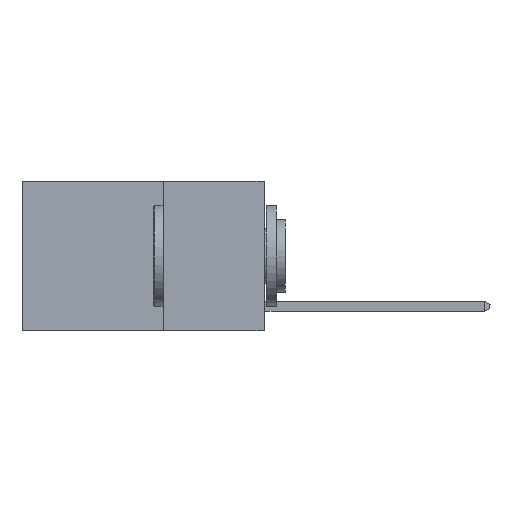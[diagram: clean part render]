
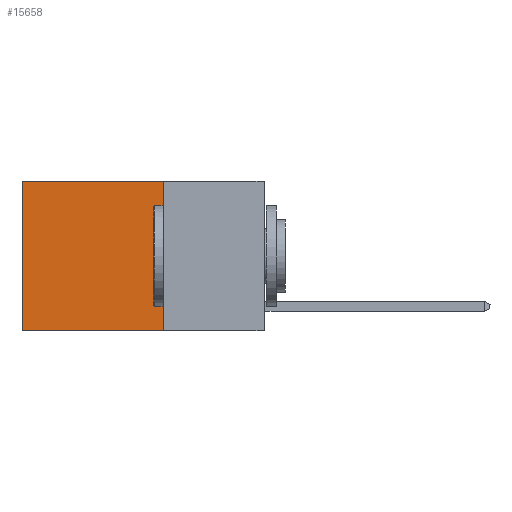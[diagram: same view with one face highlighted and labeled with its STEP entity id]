
A CAD part, left-side view. The second image highlights one B-rep face of the part: STEP entity #15658.
In plain terms, the highlighted planar face has unit normal (-1, 0, 0).
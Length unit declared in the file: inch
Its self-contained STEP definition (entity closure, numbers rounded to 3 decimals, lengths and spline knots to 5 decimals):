
#1158 = DIRECTION ( 'NONE',  ( 0., 1., 0. ) ) ;
#2014 = ORIENTED_EDGE ( 'NONE', *, *, #3535, .T. ) ;
#2140 = LINE ( 'NONE', #5242, #6266 ) ;
#3189 = LINE ( 'NONE', #15105, #11526 ) ;
#3535 = EDGE_CURVE ( 'NONE', #20967, #20801, #2140, .T. ) ;
#3891 = VECTOR ( 'NONE', #13167, 39.37008 ) ;
#5242 = CARTESIAN_POINT ( 'NONE',  ( 0.2625, 0.6, 0. ) ) ;
#5927 = ORIENTED_EDGE ( 'NONE', *, *, #17753, .F. ) ;
#6100 = ORIENTED_EDGE ( 'NONE', *, *, #11430, .T. ) ;
#6115 = FACE_OUTER_BOUND ( 'NONE', #7543, .T. ) ;
#6266 = VECTOR ( 'NONE', #21471, 39.37008 ) ;
#7543 = EDGE_LOOP ( 'NONE', ( #2014, #5927, #8857, #6100 ) ) ;
#8857 = ORIENTED_EDGE ( 'NONE', *, *, #12803, .F. ) ;
#9450 = VERTEX_POINT ( 'NONE', #15922 ) ;
#11430 = EDGE_CURVE ( 'NONE', #22941, #20967, #3189, .T. ) ;
#11526 = VECTOR ( 'NONE', #1158, 39.37008 ) ;
#12537 = VECTOR ( 'NONE', #27641, 39.37008 ) ;
#12803 = EDGE_CURVE ( 'NONE', #22941, #9450, #15642, .T. ) ;
#13167 = DIRECTION ( 'NONE',  ( 0., 0., -1. ) ) ;
#13517 = DIRECTION ( 'NONE',  ( 0., 0., -1. ) ) ;
#15105 = CARTESIAN_POINT ( 'NONE',  ( 0.2625, 0.25, 0. ) ) ;
#15642 = LINE ( 'NONE', #24773, #3891 ) ;
#15658 = ADVANCED_FACE ( 'NONE', ( #6115 ), #30054, .F. ) ;
#15907 = AXIS2_PLACEMENT_3D ( 'NONE', #25119, #25570, #13517 ) ;
#15922 = CARTESIAN_POINT ( 'NONE',  ( 0.2625, 0.25, -0.37 ) ) ;
#17753 = EDGE_CURVE ( 'NONE', #9450, #20801, #23006, .T. ) ;
#20115 = CARTESIAN_POINT ( 'NONE',  ( 0.2625, 0.6, 0. ) ) ;
#20381 = CARTESIAN_POINT ( 'NONE',  ( 0.2625, 0.25, -0.37 ) ) ;
#20801 = VERTEX_POINT ( 'NONE', #21835 ) ;
#20967 = VERTEX_POINT ( 'NONE', #20115 ) ;
#21471 = DIRECTION ( 'NONE',  ( 0., 0., -1. ) ) ;
#21603 = CARTESIAN_POINT ( 'NONE',  ( 0.2625, 0.25, 0. ) ) ;
#21835 = CARTESIAN_POINT ( 'NONE',  ( 0.2625, 0.6, -0.37 ) ) ;
#22941 = VERTEX_POINT ( 'NONE', #21603 ) ;
#23006 = LINE ( 'NONE', #20381, #12537 ) ;
#24773 = CARTESIAN_POINT ( 'NONE',  ( 0.2625, 0.25, 0. ) ) ;
#25119 = CARTESIAN_POINT ( 'NONE',  ( 0.2625, 0.25, 0. ) ) ;
#25570 = DIRECTION ( 'NONE',  ( 1., 0., 0. ) ) ;
#27641 = DIRECTION ( 'NONE',  ( 0., 1., 0. ) ) ;
#30054 = PLANE ( 'NONE',  #15907 ) ;
